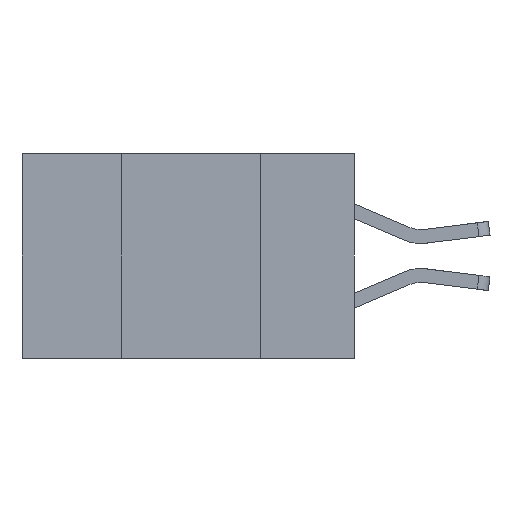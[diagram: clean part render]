
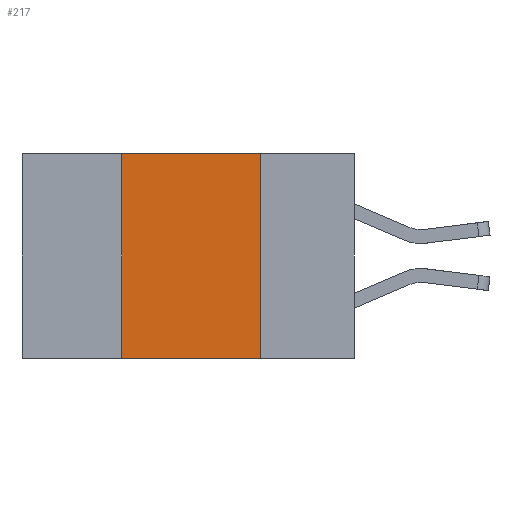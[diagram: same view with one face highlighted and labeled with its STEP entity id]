
A CAD part, left-side view. The second image highlights one B-rep face of the part: STEP entity #217.
In plain terms, the highlighted planar face has unit normal (-1, 0, 0).
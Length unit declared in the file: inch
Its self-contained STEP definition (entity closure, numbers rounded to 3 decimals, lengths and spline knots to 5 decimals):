
#172 = LINE ( 'NONE', #8970, #1943 ) ;
#217 = ADVANCED_FACE ( 'NONE', ( #6035 ), #667, .F. ) ;
#282 = EDGE_CURVE ( 'NONE', #1628, #5548, #172, .T. ) ;
#300 = VERTEX_POINT ( 'NONE', #7479 ) ;
#451 = VECTOR ( 'NONE', #9029, 39.37008 ) ;
#667 = PLANE ( 'NONE',  #8270 ) ;
#723 = CARTESIAN_POINT ( 'NONE',  ( 0., 0.42, 0. ) ) ;
#890 = ORIENTED_EDGE ( 'NONE', *, *, #7679, .F. ) ;
#1628 = VERTEX_POINT ( 'NONE', #8118 ) ;
#1759 = DIRECTION ( 'NONE',  ( 0., 0., -1. ) ) ;
#1943 = VECTOR ( 'NONE', #4363, 39.37008 ) ;
#2209 = ORIENTED_EDGE ( 'NONE', *, *, #282, .F. ) ;
#2214 = DIRECTION ( 'NONE',  ( 1., 0., 0. ) ) ;
#2262 = VECTOR ( 'NONE', #1759, 39.37008 ) ;
#2501 = CARTESIAN_POINT ( 'NONE',  ( 0., 0.17, -0.37 ) ) ;
#2504 = CARTESIAN_POINT ( 'NONE',  ( 0., 0.6, 0. ) ) ;
#2951 = CARTESIAN_POINT ( 'NONE',  ( 0., 0.6, -0.37 ) ) ;
#3527 = VERTEX_POINT ( 'NONE', #4104 ) ;
#4104 = CARTESIAN_POINT ( 'NONE',  ( 0., 0.17, 0. ) ) ;
#4124 = EDGE_CURVE ( 'NONE', #1628, #300, #9514, .T. ) ;
#4363 = DIRECTION ( 'NONE',  ( 0., 0., 1. ) ) ;
#4730 = ORIENTED_EDGE ( 'NONE', *, *, #4973, .F. ) ;
#4973 = EDGE_CURVE ( 'NONE', #3527, #300, #9078, .T. ) ;
#5373 = LINE ( 'NONE', #2504, #451 ) ;
#5548 = VERTEX_POINT ( 'NONE', #723 ) ;
#5594 = ORIENTED_EDGE ( 'NONE', *, *, #4124, .T. ) ;
#5870 = DIRECTION ( 'NONE',  ( 0., -1., 0. ) ) ;
#6035 = FACE_OUTER_BOUND ( 'NONE', #8535, .T. ) ;
#6142 = DIRECTION ( 'NONE',  ( 0., 0., -1. ) ) ;
#6850 = CARTESIAN_POINT ( 'NONE',  ( 0., 0.6, 0. ) ) ;
#7479 = CARTESIAN_POINT ( 'NONE',  ( 0., 0.17, -0.37 ) ) ;
#7679 = EDGE_CURVE ( 'NONE', #5548, #3527, #5373, .T. ) ;
#8118 = CARTESIAN_POINT ( 'NONE',  ( 0., 0.42, -0.37 ) ) ;
#8270 = AXIS2_PLACEMENT_3D ( 'NONE', #6850, #2214, #6142 ) ;
#8535 = EDGE_LOOP ( 'NONE', ( #4730, #890, #2209, #5594 ) ) ;
#8741 = VECTOR ( 'NONE', #5870, 39.37008 ) ;
#8970 = CARTESIAN_POINT ( 'NONE',  ( 0., 0.42, -0.37 ) ) ;
#9029 = DIRECTION ( 'NONE',  ( 0., -1., 0. ) ) ;
#9078 = LINE ( 'NONE', #2501, #2262 ) ;
#9514 = LINE ( 'NONE', #2951, #8741 ) ;
